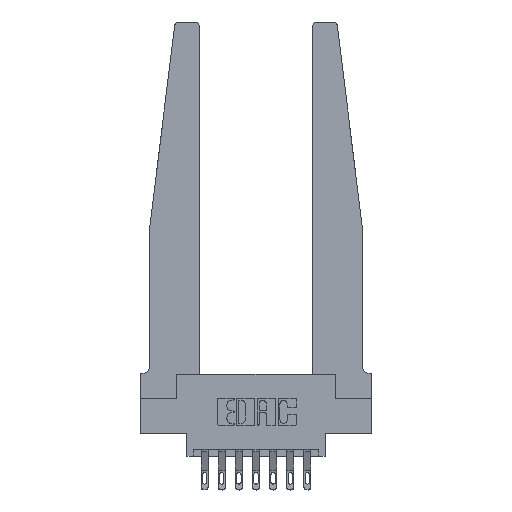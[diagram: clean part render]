
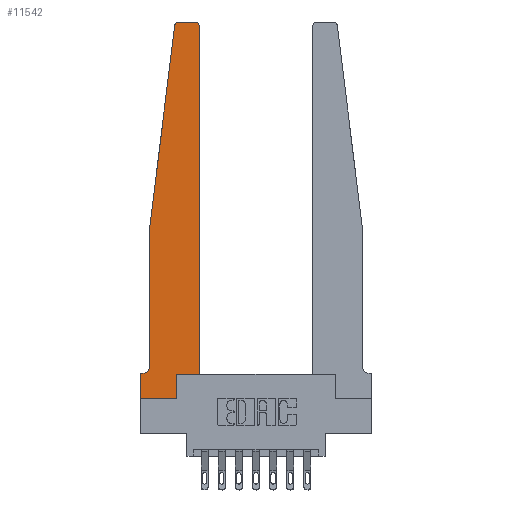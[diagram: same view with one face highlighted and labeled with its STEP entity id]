
A CAD part, top view. The second image highlights one B-rep face of the part: STEP entity #11542.
In plain terms, the highlighted planar face has unit normal (0, 0, 1).
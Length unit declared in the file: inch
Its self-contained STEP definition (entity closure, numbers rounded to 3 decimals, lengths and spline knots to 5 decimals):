
#16 = DIRECTION ( 'NONE',  ( 1., 0., 0. ) ) ;
#147 = EDGE_CURVE ( 'NONE', #13490, #14723, #6739, .T. ) ;
#281 = VECTOR ( 'NONE', #9828, 39.37008 ) ;
#588 = LINE ( 'NONE', #4085, #2062 ) ;
#629 = PLANE ( 'NONE',  #6072 ) ;
#638 = CARTESIAN_POINT ( 'NONE',  ( 0.065, 0.2375, 0.37 ) ) ;
#1161 = DIRECTION ( 'NONE',  ( 0., 0., -1. ) ) ;
#1222 = VECTOR ( 'NONE', #13168, 39.37008 ) ;
#1301 = DIRECTION ( 'NONE',  ( -1., 0., 0. ) ) ;
#1568 = VERTEX_POINT ( 'NONE', #1793 ) ;
#1585 = CARTESIAN_POINT ( 'NONE',  ( 0.2605, 0.18, 0.37 ) ) ;
#1758 = ORIENTED_EDGE ( 'NONE', *, *, #10709, .T. ) ;
#1763 = FACE_OUTER_BOUND ( 'NONE', #12152, .T. ) ;
#1793 = CARTESIAN_POINT ( 'NONE',  ( 0.395, 2.75, 0.37 ) ) ;
#1828 = ORIENTED_EDGE ( 'NONE', *, *, #9109, .T. ) ;
#1872 = CARTESIAN_POINT ( 'NONE',  ( 0., 0.1875, 0.37 ) ) ;
#2011 = CARTESIAN_POINT ( 'NONE',  ( 0.065, 1.25, 0.37 ) ) ;
#2062 = VECTOR ( 'NONE', #2947, 39.37008 ) ;
#2140 = EDGE_CURVE ( 'NONE', #5084, #5871, #12376, .T. ) ;
#2151 = DIRECTION ( 'NONE',  ( 1., 0., 0. ) ) ;
#2683 = EDGE_CURVE ( 'NONE', #11498, #1568, #14030, .T. ) ;
#2945 = CARTESIAN_POINT ( 'NONE',  ( 0.425, 0.18, 0.37 ) ) ;
#2947 = DIRECTION ( 'NONE',  ( 0., -1., 0. ) ) ;
#3138 = VECTOR ( 'NONE', #12329, 39.37008 ) ;
#3392 = CARTESIAN_POINT ( 'NONE',  ( 0.2605, 0., 0.37 ) ) ;
#3577 = VERTEX_POINT ( 'NONE', #638 ) ;
#4085 = CARTESIAN_POINT ( 'NONE',  ( 0., 0., 0.37 ) ) ;
#4129 = EDGE_CURVE ( 'NONE', #5871, #3577, #5456, .T. ) ;
#4158 = CARTESIAN_POINT ( 'NONE',  ( 0., 0., 0.37 ) ) ;
#4331 = EDGE_CURVE ( 'NONE', #9496, #5241, #588, .T. ) ;
#4650 = DIRECTION ( 'NONE',  ( -1., 0., 0. ) ) ;
#4658 = AXIS2_PLACEMENT_3D ( 'NONE', #9092, #13555, #16 ) ;
#4924 = ORIENTED_EDGE ( 'NONE', *, *, #10454, .T. ) ;
#5084 = VERTEX_POINT ( 'NONE', #7927 ) ;
#5173 = DIRECTION ( 'NONE',  ( -1., 0., 0. ) ) ;
#5220 = LINE ( 'NONE', #4158, #281 ) ;
#5241 = VERTEX_POINT ( 'NONE', #14046 ) ;
#5456 = LINE ( 'NONE', #14678, #9775 ) ;
#5550 = CARTESIAN_POINT ( 'NONE',  ( 0.395, 2.72, 0.37 ) ) ;
#5801 = CARTESIAN_POINT ( 'NONE',  ( 0.425, 0.18, 0.37 ) ) ;
#5871 = VERTEX_POINT ( 'NONE', #14734 ) ;
#5892 = CIRCLE ( 'NONE', #4658, 0.03 ) ;
#6072 = AXIS2_PLACEMENT_3D ( 'NONE', #7666, #11519, #12426 ) ;
#6143 = ORIENTED_EDGE ( 'NONE', *, *, #147, .T. ) ;
#6197 = VECTOR ( 'NONE', #5173, 39.37008 ) ;
#6313 = CARTESIAN_POINT ( 'NONE',  ( 0.065, 0.1875, 0.37 ) ) ;
#6348 = CARTESIAN_POINT ( 'NONE',  ( 0.2605, 0.18, 0.37 ) ) ;
#6454 = ORIENTED_EDGE ( 'NONE', *, *, #2683, .T. ) ;
#6496 = CARTESIAN_POINT ( 'NONE',  ( 0.27653, 2.75, 0.37 ) ) ;
#6544 = ORIENTED_EDGE ( 'NONE', *, *, #2140, .T. ) ;
#6739 = LINE ( 'NONE', #11347, #3138 ) ;
#6764 = CARTESIAN_POINT ( 'NONE',  ( 0.25, 2.75, 0.37 ) ) ;
#6884 = AXIS2_PLACEMENT_3D ( 'NONE', #11532, #1161, #4650 ) ;
#7020 = EDGE_CURVE ( 'NONE', #1568, #7693, #13791, .T. ) ;
#7054 = ORIENTED_EDGE ( 'NONE', *, *, #9671, .T. ) ;
#7485 = CARTESIAN_POINT ( 'NONE',  ( 0.015, 0.1875, 0.37 ) ) ;
#7553 = ORIENTED_EDGE ( 'NONE', *, *, #12553, .T. ) ;
#7666 = CARTESIAN_POINT ( 'NONE',  ( 0., 0.1875, 0.37 ) ) ;
#7693 = VERTEX_POINT ( 'NONE', #6496 ) ;
#7927 = CARTESIAN_POINT ( 'NONE',  ( 0.24675, 2.72367, 0.37 ) ) ;
#7967 = VECTOR ( 'NONE', #8962, 39.37008 ) ;
#8355 = VECTOR ( 'NONE', #1301, 39.37008 ) ;
#8962 = DIRECTION ( 'NONE',  ( -0.122, -0.992, 0. ) ) ;
#9092 = CARTESIAN_POINT ( 'NONE',  ( 0.27653, 2.72, 0.37 ) ) ;
#9109 = EDGE_CURVE ( 'NONE', #5241, #13516, #5220, .T. ) ;
#9496 = VERTEX_POINT ( 'NONE', #1872 ) ;
#9671 = EDGE_CURVE ( 'NONE', #3577, #13440, #10257, .T. ) ;
#9775 = VECTOR ( 'NONE', #12575, 39.37008 ) ;
#9828 = DIRECTION ( 'NONE',  ( 1., 0., 0. ) ) ;
#10152 = AXIS2_PLACEMENT_3D ( 'NONE', #5550, #12515, #2151 ) ;
#10257 = CIRCLE ( 'NONE', #6884, 0.05 ) ;
#10454 = EDGE_CURVE ( 'NONE', #7693, #5084, #5892, .T. ) ;
#10709 = EDGE_CURVE ( 'NONE', #13516, #13490, #11955, .T. ) ;
#10744 = ORIENTED_EDGE ( 'NONE', *, *, #7020, .T. ) ;
#11347 = CARTESIAN_POINT ( 'NONE',  ( 0.425, 0.18, 0.37 ) ) ;
#11381 = ORIENTED_EDGE ( 'NONE', *, *, #4331, .T. ) ;
#11498 = VERTEX_POINT ( 'NONE', #13339 ) ;
#11519 = DIRECTION ( 'NONE',  ( 0., 0., 1. ) ) ;
#11532 = CARTESIAN_POINT ( 'NONE',  ( 0.015, 0.2375, 0.37 ) ) ;
#11542 = ADVANCED_FACE ( 'NONE', ( #1763 ), #629, .T. ) ;
#11940 = LINE ( 'NONE', #2945, #13233 ) ;
#11955 = LINE ( 'NONE', #1585, #1222 ) ;
#12152 = EDGE_LOOP ( 'NONE', ( #10744, #4924, #6544, #13584, #7054, #7553, #11381, #1828, #1758, #6143, #12326, #6454 ) ) ;
#12171 = DIRECTION ( 'NONE',  ( 0., 1., 0. ) ) ;
#12326 = ORIENTED_EDGE ( 'NONE', *, *, #14109, .T. ) ;
#12329 = DIRECTION ( 'NONE',  ( 1., 0., 0. ) ) ;
#12376 = LINE ( 'NONE', #2011, #7967 ) ;
#12426 = DIRECTION ( 'NONE',  ( 1., 0., 0. ) ) ;
#12515 = DIRECTION ( 'NONE',  ( 0., 0., 1. ) ) ;
#12553 = EDGE_CURVE ( 'NONE', #13440, #9496, #13488, .T. ) ;
#12575 = DIRECTION ( 'NONE',  ( 0., -1., 0. ) ) ;
#13168 = DIRECTION ( 'NONE',  ( 0., 1., 0. ) ) ;
#13233 = VECTOR ( 'NONE', #12171, 39.37008 ) ;
#13339 = CARTESIAN_POINT ( 'NONE',  ( 0.425, 2.72, 0.37 ) ) ;
#13440 = VERTEX_POINT ( 'NONE', #7485 ) ;
#13488 = LINE ( 'NONE', #6313, #6197 ) ;
#13490 = VERTEX_POINT ( 'NONE', #6348 ) ;
#13516 = VERTEX_POINT ( 'NONE', #3392 ) ;
#13555 = DIRECTION ( 'NONE',  ( 0., 0., 1. ) ) ;
#13584 = ORIENTED_EDGE ( 'NONE', *, *, #4129, .T. ) ;
#13791 = LINE ( 'NONE', #6764, #8355 ) ;
#14030 = CIRCLE ( 'NONE', #10152, 0.03 ) ;
#14046 = CARTESIAN_POINT ( 'NONE',  ( 0., 0., 0.37 ) ) ;
#14109 = EDGE_CURVE ( 'NONE', #14723, #11498, #11940, .T. ) ;
#14678 = CARTESIAN_POINT ( 'NONE',  ( 0.065, 1.25, 0.37 ) ) ;
#14723 = VERTEX_POINT ( 'NONE', #5801 ) ;
#14734 = CARTESIAN_POINT ( 'NONE',  ( 0.065, 1.25, 0.37 ) ) ;
